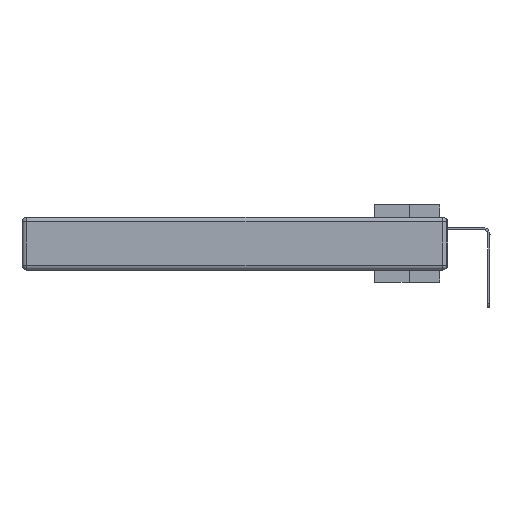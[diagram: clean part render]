
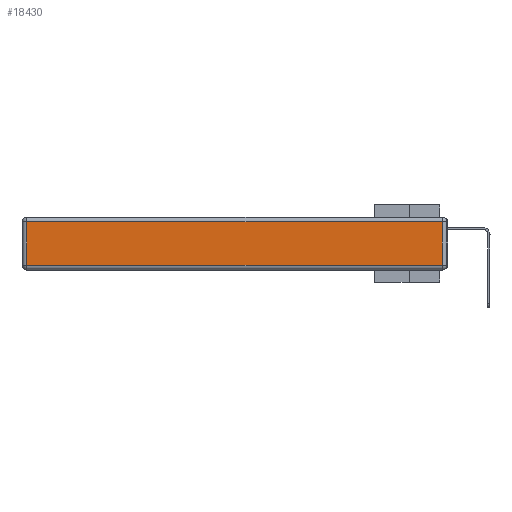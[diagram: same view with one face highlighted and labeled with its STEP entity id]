
A CAD part, left-side view. The second image highlights one B-rep face of the part: STEP entity #18430.
In plain terms, the highlighted planar face has unit normal (-1, 0, 0).
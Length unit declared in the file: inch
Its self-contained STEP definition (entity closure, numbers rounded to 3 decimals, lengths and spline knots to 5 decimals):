
#30 = EDGE_CURVE ( 'NONE', #3013, #14660, #9673, .T. ) ;
#2013 = LINE ( 'NONE', #4259, #19090 ) ;
#3013 = VERTEX_POINT ( 'NONE', #5916 ) ;
#4259 = CARTESIAN_POINT ( 'NONE',  ( 0., 0., -0.313 ) ) ;
#5767 = ORIENTED_EDGE ( 'NONE', *, *, #19894, .T. ) ;
#5916 = CARTESIAN_POINT ( 'NONE',  ( 0., 0.03, -0.03 ) ) ;
#5975 = VECTOR ( 'NONE', #8248, 39.37008 ) ;
#6620 = VERTEX_POINT ( 'NONE', #10408 ) ;
#8248 = DIRECTION ( 'NONE',  ( 0., 0., -1. ) ) ;
#8576 = DIRECTION ( 'NONE',  ( 0., 0., 1. ) ) ;
#9673 = LINE ( 'NONE', #29639, #29191 ) ;
#10408 = CARTESIAN_POINT ( 'NONE',  ( 0., 2.72, -0.313 ) ) ;
#10956 = CARTESIAN_POINT ( 'NONE',  ( 0., 0.03, -0.343 ) ) ;
#11213 = PLANE ( 'NONE',  #19014 ) ;
#13772 = DIRECTION ( 'NONE',  ( -1., 0., 0. ) ) ;
#14519 = LINE ( 'NONE', #10956, #24896 ) ;
#14660 = VERTEX_POINT ( 'NONE', #24915 ) ;
#14992 = EDGE_CURVE ( 'NONE', #20033, #3013, #14519, .T. ) ;
#16467 = ORIENTED_EDGE ( 'NONE', *, *, #14992, .T. ) ;
#17226 = EDGE_CURVE ( 'NONE', #14660, #6620, #24314, .T. ) ;
#18430 = ADVANCED_FACE ( 'NONE', ( #30833 ), #11213, .T. ) ;
#18605 = DIRECTION ( 'NONE',  ( 0., 0., 1. ) ) ;
#19014 = AXIS2_PLACEMENT_3D ( 'NONE', #29374, #13772, #8576 ) ;
#19090 = VECTOR ( 'NONE', #27291, 39.37008 ) ;
#19894 = EDGE_CURVE ( 'NONE', #6620, #20033, #2013, .T. ) ;
#20033 = VERTEX_POINT ( 'NONE', #25181 ) ;
#21955 = DIRECTION ( 'NONE',  ( 0., 1., 0. ) ) ;
#24314 = LINE ( 'NONE', #25308, #5975 ) ;
#24491 = ORIENTED_EDGE ( 'NONE', *, *, #17226, .T. ) ;
#24674 = EDGE_LOOP ( 'NONE', ( #5767, #16467, #30399, #24491 ) ) ;
#24896 = VECTOR ( 'NONE', #18605, 39.37008 ) ;
#24915 = CARTESIAN_POINT ( 'NONE',  ( 0., 2.72, -0.03 ) ) ;
#25181 = CARTESIAN_POINT ( 'NONE',  ( 0., 0.03, -0.313 ) ) ;
#25308 = CARTESIAN_POINT ( 'NONE',  ( 0., 2.72, -0.343 ) ) ;
#27291 = DIRECTION ( 'NONE',  ( 0., -1., 0. ) ) ;
#29191 = VECTOR ( 'NONE', #21955, 39.37008 ) ;
#29374 = CARTESIAN_POINT ( 'NONE',  ( 0., 0., -0.343 ) ) ;
#29639 = CARTESIAN_POINT ( 'NONE',  ( 0., 2.75, -0.03 ) ) ;
#30399 = ORIENTED_EDGE ( 'NONE', *, *, #30, .T. ) ;
#30833 = FACE_OUTER_BOUND ( 'NONE', #24674, .T. ) ;
